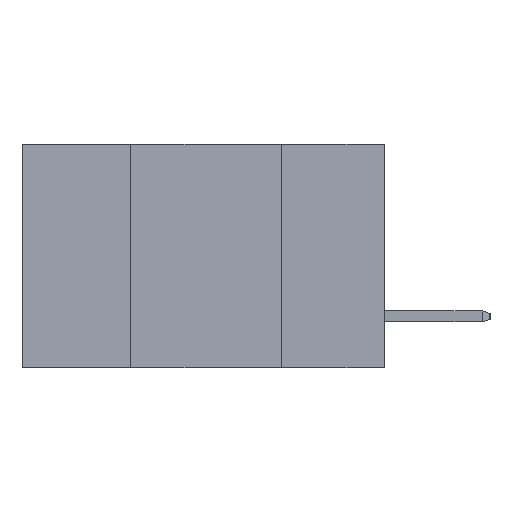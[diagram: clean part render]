
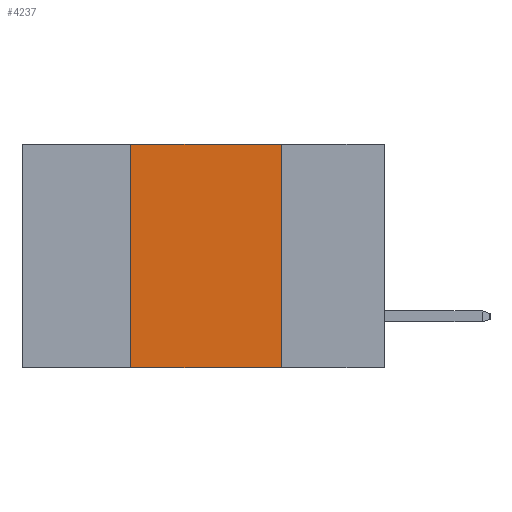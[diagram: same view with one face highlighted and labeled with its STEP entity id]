
A CAD part, left-side view. The second image highlights one B-rep face of the part: STEP entity #4237.
In plain terms, the highlighted planar face has unit normal (-1, 0, 0).
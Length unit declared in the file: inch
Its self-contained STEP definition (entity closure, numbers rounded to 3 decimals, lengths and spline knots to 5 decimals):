
#67 = DIRECTION ( 'NONE',  ( 0., 0., -1. ) ) ;
#1878 = VERTEX_POINT ( 'NONE', #11158 ) ;
#2155 = AXIS2_PLACEMENT_3D ( 'NONE', #4103, #18797, #9957 ) ;
#2513 = LINE ( 'NONE', #3224, #17728 ) ;
#3224 = CARTESIAN_POINT ( 'NONE',  ( 0., 0.6, 0. ) ) ;
#3269 = EDGE_CURVE ( 'NONE', #16559, #1878, #5617, .T. ) ;
#3823 = ORIENTED_EDGE ( 'NONE', *, *, #11862, .F. ) ;
#4103 = CARTESIAN_POINT ( 'NONE',  ( 0., 0.6, 0. ) ) ;
#4237 = ADVANCED_FACE ( 'NONE', ( #11231 ), #8508, .F. ) ;
#5617 = LINE ( 'NONE', #8427, #6535 ) ;
#5819 = VECTOR ( 'NONE', #67, 39.37008 ) ;
#6015 = CARTESIAN_POINT ( 'NONE',  ( 0., 0.17, 0. ) ) ;
#6535 = VECTOR ( 'NONE', #8494, 39.37008 ) ;
#6724 = CARTESIAN_POINT ( 'NONE',  ( 0., 0.42, -0.37 ) ) ;
#7111 = VECTOR ( 'NONE', #18008, 39.37008 ) ;
#8427 = CARTESIAN_POINT ( 'NONE',  ( 0., 0.42, 0. ) ) ;
#8494 = DIRECTION ( 'NONE',  ( 0., 0., 1. ) ) ;
#8508 = PLANE ( 'NONE',  #2155 ) ;
#9178 = CARTESIAN_POINT ( 'NONE',  ( 0., 0.6, -0.37 ) ) ;
#9957 = DIRECTION ( 'NONE',  ( 0., 0., -1. ) ) ;
#10514 = DIRECTION ( 'NONE',  ( 0., -1., 0. ) ) ;
#11158 = CARTESIAN_POINT ( 'NONE',  ( 0., 0.42, 0. ) ) ;
#11226 = ORIENTED_EDGE ( 'NONE', *, *, #3269, .F. ) ;
#11231 = FACE_OUTER_BOUND ( 'NONE', #16440, .T. ) ;
#11430 = LINE ( 'NONE', #9178, #7111 ) ;
#11829 = CARTESIAN_POINT ( 'NONE',  ( 0., 0.17, -0.37 ) ) ;
#11862 = EDGE_CURVE ( 'NONE', #15156, #18197, #13135, .T. ) ;
#12620 = EDGE_CURVE ( 'NONE', #1878, #15156, #2513, .T. ) ;
#13135 = LINE ( 'NONE', #6015, #5819 ) ;
#13137 = EDGE_CURVE ( 'NONE', #16559, #18197, #11430, .T. ) ;
#13284 = ORIENTED_EDGE ( 'NONE', *, *, #12620, .F. ) ;
#13869 = CARTESIAN_POINT ( 'NONE',  ( 0., 0.17, 0. ) ) ;
#15156 = VERTEX_POINT ( 'NONE', #13869 ) ;
#16440 = EDGE_LOOP ( 'NONE', ( #3823, #13284, #11226, #18093 ) ) ;
#16559 = VERTEX_POINT ( 'NONE', #6724 ) ;
#17728 = VECTOR ( 'NONE', #10514, 39.37008 ) ;
#18008 = DIRECTION ( 'NONE',  ( 0., -1., 0. ) ) ;
#18093 = ORIENTED_EDGE ( 'NONE', *, *, #13137, .T. ) ;
#18197 = VERTEX_POINT ( 'NONE', #11829 ) ;
#18797 = DIRECTION ( 'NONE',  ( 1., 0., 0. ) ) ;
